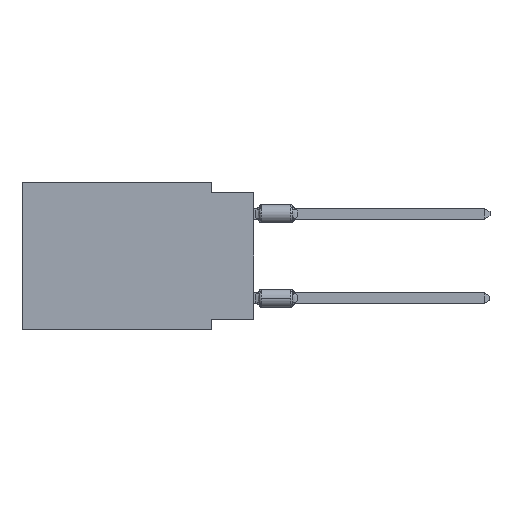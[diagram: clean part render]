
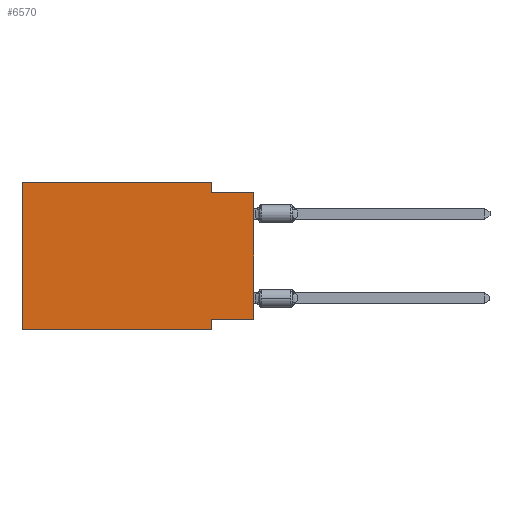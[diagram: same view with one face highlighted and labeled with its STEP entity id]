
A CAD part, left-side view. The second image highlights one B-rep face of the part: STEP entity #6570.
In plain terms, the highlighted planar face has unit normal (-1, 0, 0).
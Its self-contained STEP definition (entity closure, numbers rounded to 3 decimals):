
#959 = VECTOR ( 'NONE', #17356, 1000. ) ;
#1404 = LINE ( 'NONE', #34979, #22134 ) ;
#1921 = LINE ( 'NONE', #24564, #18084 ) ;
#2764 = LINE ( 'NONE', #17247, #7926 ) ;
#3331 = FACE_OUTER_BOUND ( 'NONE', #10624, .T. ) ;
#3617 = CARTESIAN_POINT ( 'NONE',  ( 0., 2.54, 0. ) ) ;
#3745 = EDGE_CURVE ( 'NONE', #12274, #12321, #1404, .T. ) ;
#3819 = CARTESIAN_POINT ( 'NONE',  ( 0., 2.54, -8.255 ) ) ;
#4019 = DIRECTION ( 'NONE',  ( 0., 0., 1. ) ) ;
#4982 = CARTESIAN_POINT ( 'NONE',  ( 0., 0., -0.635 ) ) ;
#5233 = EDGE_CURVE ( 'NONE', #17217, #23912, #36633, .T. ) ;
#6204 = CARTESIAN_POINT ( 'NONE',  ( 0., 13.97, -8.89 ) ) ;
#6300 = CARTESIAN_POINT ( 'NONE',  ( 0., 13.97, 0. ) ) ;
#6570 = ADVANCED_FACE ( 'NONE', ( #3331 ), #31713, .F. ) ;
#7062 = ORIENTED_EDGE ( 'NONE', *, *, #8556, .F. ) ;
#7926 = VECTOR ( 'NONE', #14274, 1000. ) ;
#8556 = EDGE_CURVE ( 'NONE', #27079, #9580, #31266, .T. ) ;
#9007 = CARTESIAN_POINT ( 'NONE',  ( 0., 2.54, -8.89 ) ) ;
#9580 = VERTEX_POINT ( 'NONE', #20969 ) ;
#10463 = DIRECTION ( 'NONE',  ( 0., 1., 0. ) ) ;
#10624 = EDGE_LOOP ( 'NONE', ( #19396, #11944, #30062, #21392, #21793, #22682, #7062, #36617 ) ) ;
#11061 = VECTOR ( 'NONE', #13723, 1000. ) ;
#11944 = ORIENTED_EDGE ( 'NONE', *, *, #24584, .F. ) ;
#12148 = DIRECTION ( 'NONE',  ( 0., -1., 0. ) ) ;
#12274 = VERTEX_POINT ( 'NONE', #36403 ) ;
#12321 = VERTEX_POINT ( 'NONE', #35081 ) ;
#13723 = DIRECTION ( 'NONE',  ( 0., -1., 0. ) ) ;
#14274 = DIRECTION ( 'NONE',  ( 0., 0., 1. ) ) ;
#14524 = EDGE_CURVE ( 'NONE', #17972, #9580, #22913, .T. ) ;
#14667 = AXIS2_PLACEMENT_3D ( 'NONE', #6300, #17633, #28941 ) ;
#15255 = CARTESIAN_POINT ( 'NONE',  ( 0., 13.97, 0. ) ) ;
#15605 = VERTEX_POINT ( 'NONE', #22735 ) ;
#16381 = EDGE_CURVE ( 'NONE', #15605, #17217, #18580, .T. ) ;
#16497 = LINE ( 'NONE', #4982, #11061 ) ;
#17217 = VERTEX_POINT ( 'NONE', #35667 ) ;
#17247 = CARTESIAN_POINT ( 'NONE',  ( 0., 13.97, 0. ) ) ;
#17356 = DIRECTION ( 'NONE',  ( 0., 0., -1. ) ) ;
#17633 = DIRECTION ( 'NONE',  ( 1., 0., 0. ) ) ;
#17972 = VERTEX_POINT ( 'NONE', #18542 ) ;
#18084 = VECTOR ( 'NONE', #10463, 1000. ) ;
#18542 = CARTESIAN_POINT ( 'NONE',  ( 0., 13.97, -8.89 ) ) ;
#18580 = LINE ( 'NONE', #15255, #25893 ) ;
#18765 = DIRECTION ( 'NONE',  ( 0., -1., 0. ) ) ;
#19396 = ORIENTED_EDGE ( 'NONE', *, *, #3745, .T. ) ;
#20969 = CARTESIAN_POINT ( 'NONE',  ( 0., 2.54, -8.89 ) ) ;
#21392 = ORIENTED_EDGE ( 'NONE', *, *, #16381, .F. ) ;
#21793 = ORIENTED_EDGE ( 'NONE', *, *, #25902, .F. ) ;
#22134 = VECTOR ( 'NONE', #4019, 1000. ) ;
#22596 = EDGE_CURVE ( 'NONE', #12274, #27079, #1921, .T. ) ;
#22682 = ORIENTED_EDGE ( 'NONE', *, *, #14524, .T. ) ;
#22735 = CARTESIAN_POINT ( 'NONE',  ( 0., 13.97, 0. ) ) ;
#22913 = LINE ( 'NONE', #6204, #27552 ) ;
#23912 = VERTEX_POINT ( 'NONE', #28806 ) ;
#24564 = CARTESIAN_POINT ( 'NONE',  ( 0., 0., -8.255 ) ) ;
#24584 = EDGE_CURVE ( 'NONE', #23912, #12321, #16497, .T. ) ;
#25893 = VECTOR ( 'NONE', #18765, 1000. ) ;
#25902 = EDGE_CURVE ( 'NONE', #17972, #15605, #2764, .T. ) ;
#27079 = VERTEX_POINT ( 'NONE', #3819 ) ;
#27552 = VECTOR ( 'NONE', #12148, 1000. ) ;
#28806 = CARTESIAN_POINT ( 'NONE',  ( 0., 2.54, -0.635 ) ) ;
#28941 = DIRECTION ( 'NONE',  ( 0., 0., -1. ) ) ;
#30062 = ORIENTED_EDGE ( 'NONE', *, *, #5233, .F. ) ;
#31266 = LINE ( 'NONE', #9007, #35480 ) ;
#31713 = PLANE ( 'NONE',  #14667 ) ;
#34767 = DIRECTION ( 'NONE',  ( 0., 0., -1. ) ) ;
#34979 = CARTESIAN_POINT ( 'NONE',  ( 0., 0., 0. ) ) ;
#35081 = CARTESIAN_POINT ( 'NONE',  ( 0., 0., -0.635 ) ) ;
#35480 = VECTOR ( 'NONE', #34767, 1000. ) ;
#35667 = CARTESIAN_POINT ( 'NONE',  ( 0., 2.54, 0. ) ) ;
#36403 = CARTESIAN_POINT ( 'NONE',  ( 0., 0., -8.255 ) ) ;
#36617 = ORIENTED_EDGE ( 'NONE', *, *, #22596, .F. ) ;
#36633 = LINE ( 'NONE', #3617, #959 ) ;
